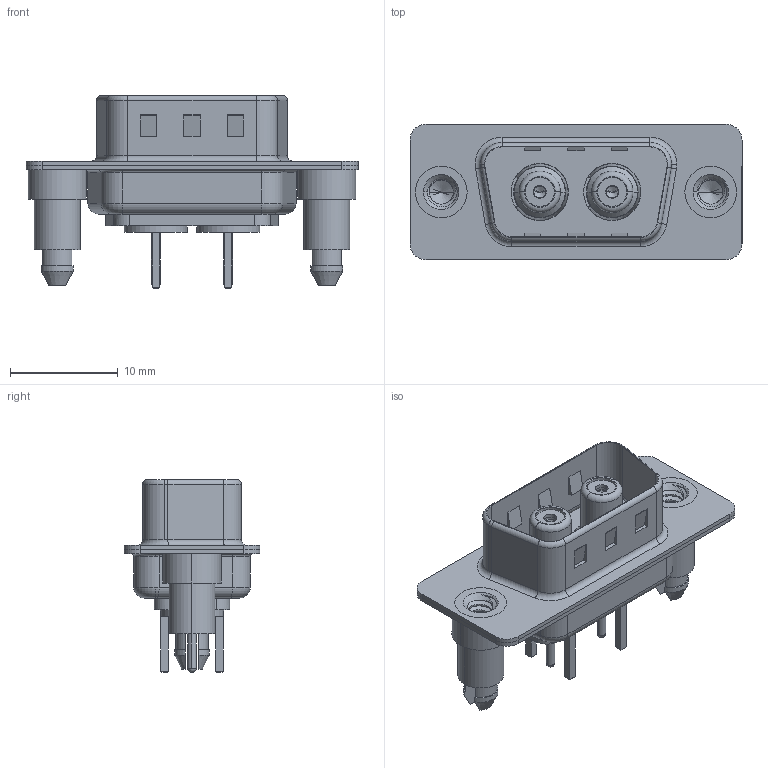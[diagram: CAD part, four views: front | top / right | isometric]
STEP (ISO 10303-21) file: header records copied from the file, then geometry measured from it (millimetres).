
FILE_DESCRIPTION (( 'STEP AP203' ), '1' );
FILE_NAME ('627-2W2-624-5T5.STEP', '2019-05-23T23:32:07', ( '' ), ( '' ), 'SwSTEP 2.0', 'SolidWorks 2016', '' );
FILE_SCHEMA (( 'CONFIG_CONTROL_DESIGN' ));
Length unit declared in the file: millimetre
Products named in the file (11): Locking Collar; Socket_Str; Co-Ax Jack Assy_S; 627-2W2-624-5T5; 627Combo Housing_2W2; 627Combo Threaded Boardlock_5; 627Combo Shell Rear_09 Contacts; Co-Ax Jack_Straight PC Tail; 627Combo Shell Front_09 Contacts; Insulator Socket; Insulator Socket 2
Assembly tree (12 placements, depth 3):
  627-2W2-624-5T5
    627Combo Housing_2W2
    627Combo Shell Rear_09 Contacts
    627Combo Shell Front_09 Contacts
    627Combo Threaded Boardlock_5  x2
    Co-Ax Jack Assy_S  x2
      Co-Ax Jack_Straight PC Tail
      Insulator Socket
      Insulator Socket 2
      Locking Collar
      Socket_Str
Bounding box: 30.8 x 12.6 x 17.9 mm (x, y, z)
Volume: 1491.3 mm3; surface area: 4733.9 mm2
Topology: 15 solids, 15 shells, 576 faces, 1387 edges, 872 vertices
Faces by surface type: cylinder 255, plane 217, torus 58, cone 32, bspline 10, sphere 4
Entity records: 14982 total; most frequent: CARTESIAN_POINT 3908, DIRECTION 2168, ORIENTED_EDGE 1990, EDGE_CURVE 995, AXIS2_PLACEMENT_3D 834, VERTEX_POINT 629, LINE 500, VECTOR 500
